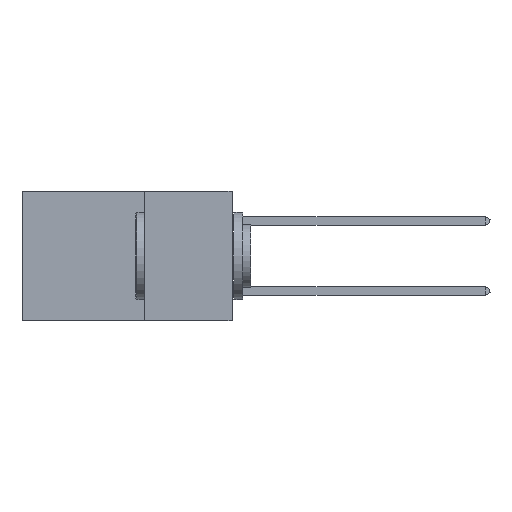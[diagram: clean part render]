
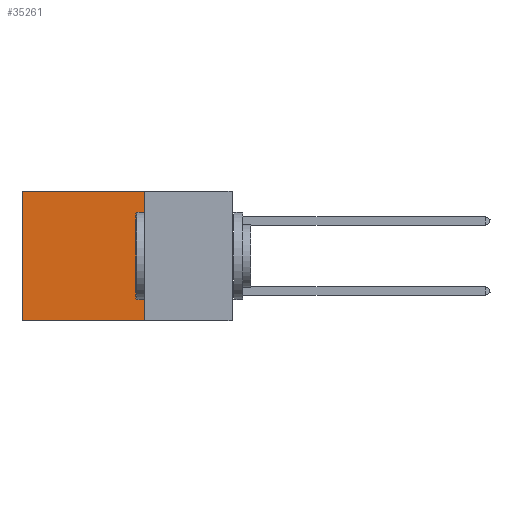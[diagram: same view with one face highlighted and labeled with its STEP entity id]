
A CAD part, left-side view. The second image highlights one B-rep face of the part: STEP entity #35261.
In plain terms, the highlighted planar face has unit normal (-1, 0, 0).
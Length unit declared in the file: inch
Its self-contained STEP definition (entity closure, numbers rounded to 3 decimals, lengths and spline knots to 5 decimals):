
#1153 = VERTEX_POINT ( 'NONE', #6095 ) ;
#2215 = DIRECTION ( 'NONE',  ( 0., 1., 0. ) ) ;
#2396 = VERTEX_POINT ( 'NONE', #2706 ) ;
#2706 = CARTESIAN_POINT ( 'NONE',  ( 0.2875, 0.6, 0. ) ) ;
#4631 = DIRECTION ( 'NONE',  ( 1., 0., 0. ) ) ;
#5187 = EDGE_CURVE ( 'NONE', #2396, #1153, #13289, .T. ) ;
#6095 = CARTESIAN_POINT ( 'NONE',  ( 0.2875, 0.6, -0.37 ) ) ;
#6367 = FACE_OUTER_BOUND ( 'NONE', #12906, .T. ) ;
#8135 = LINE ( 'NONE', #34322, #39337 ) ;
#9217 = EDGE_CURVE ( 'NONE', #14641, #1153, #8135, .T. ) ;
#9312 = ORIENTED_EDGE ( 'NONE', *, *, #30053, .F. ) ;
#11323 = DIRECTION ( 'NONE',  ( 0., 0., -1. ) ) ;
#12906 = EDGE_LOOP ( 'NONE', ( #25749, #39452, #9312, #13808 ) ) ;
#13289 = LINE ( 'NONE', #29490, #37270 ) ;
#13808 = ORIENTED_EDGE ( 'NONE', *, *, #32639, .T. ) ;
#14423 = VECTOR ( 'NONE', #33483, 39.37008 ) ;
#14641 = VERTEX_POINT ( 'NONE', #20795 ) ;
#15395 = LINE ( 'NONE', #39290, #14423 ) ;
#17002 = PLANE ( 'NONE',  #30312 ) ;
#20795 = CARTESIAN_POINT ( 'NONE',  ( 0.2875, 0.25, -0.37 ) ) ;
#21567 = VERTEX_POINT ( 'NONE', #32540 ) ;
#23069 = CARTESIAN_POINT ( 'NONE',  ( 0.2875, 0.25, 0. ) ) ;
#25749 = ORIENTED_EDGE ( 'NONE', *, *, #5187, .T. ) ;
#26098 = DIRECTION ( 'NONE',  ( 0., 0., -1. ) ) ;
#28859 = LINE ( 'NONE', #32610, #35867 ) ;
#29490 = CARTESIAN_POINT ( 'NONE',  ( 0.2875, 0.6, 0. ) ) ;
#30053 = EDGE_CURVE ( 'NONE', #21567, #14641, #15395, .T. ) ;
#30312 = AXIS2_PLACEMENT_3D ( 'NONE', #23069, #4631, #26098 ) ;
#32540 = CARTESIAN_POINT ( 'NONE',  ( 0.2875, 0.25, 0. ) ) ;
#32610 = CARTESIAN_POINT ( 'NONE',  ( 0.2875, 0.25, 0. ) ) ;
#32639 = EDGE_CURVE ( 'NONE', #21567, #2396, #28859, .T. ) ;
#33483 = DIRECTION ( 'NONE',  ( 0., 0., -1. ) ) ;
#34322 = CARTESIAN_POINT ( 'NONE',  ( 0.2875, 0.25, -0.37 ) ) ;
#35261 = ADVANCED_FACE ( 'NONE', ( #6367 ), #17002, .F. ) ;
#35867 = VECTOR ( 'NONE', #2215, 39.37008 ) ;
#37270 = VECTOR ( 'NONE', #11323, 39.37008 ) ;
#37295 = DIRECTION ( 'NONE',  ( 0., 1., 0. ) ) ;
#39290 = CARTESIAN_POINT ( 'NONE',  ( 0.2875, 0.25, 0. ) ) ;
#39337 = VECTOR ( 'NONE', #37295, 39.37008 ) ;
#39452 = ORIENTED_EDGE ( 'NONE', *, *, #9217, .F. ) ;
